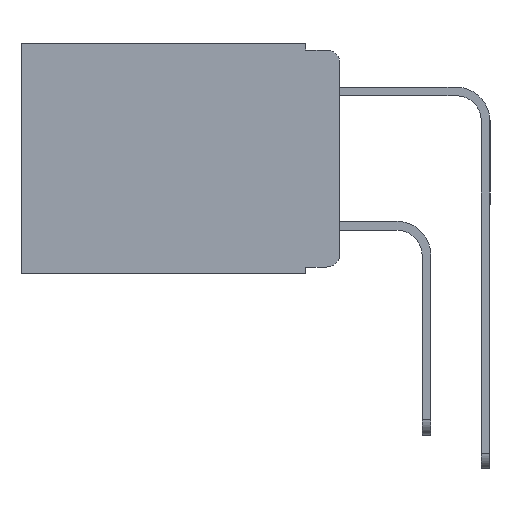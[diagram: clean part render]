
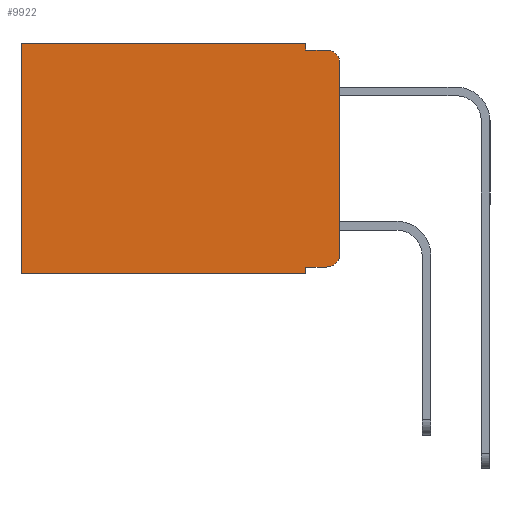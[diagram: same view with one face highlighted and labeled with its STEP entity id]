
A CAD part, left-side view. The second image highlights one B-rep face of the part: STEP entity #9922.
In plain terms, the highlighted planar face has unit normal (-1, 0, 0).
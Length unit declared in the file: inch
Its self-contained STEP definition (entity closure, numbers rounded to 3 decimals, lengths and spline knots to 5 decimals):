
#86 = DIRECTION ( 'NONE',  ( 0., -1., 0. ) ) ;
#463 = ORIENTED_EDGE ( 'NONE', *, *, #11980, .T. ) ;
#1903 = ORIENTED_EDGE ( 'NONE', *, *, #7288, .F. ) ;
#2414 = DIRECTION ( 'NONE',  ( 0., 1., 0. ) ) ;
#2755 = DIRECTION ( 'NONE',  ( 0., -1., 0. ) ) ;
#2843 = PLANE ( 'NONE',  #14372 ) ;
#3062 = VERTEX_POINT ( 'NONE', #25714 ) ;
#3733 = CARTESIAN_POINT ( 'NONE',  ( 0.298, 0.02, -0.01 ) ) ;
#3858 = CIRCLE ( 'NONE', #24096, 0.02 ) ;
#4235 = DIRECTION ( 'NONE',  ( -1., 0., 0. ) ) ;
#4253 = DIRECTION ( 'NONE',  ( 0., 1., 0. ) ) ;
#4342 = LINE ( 'NONE', #17061, #10380 ) ;
#4482 = ORIENTED_EDGE ( 'NONE', *, *, #24806, .T. ) ;
#4807 = CARTESIAN_POINT ( 'NONE',  ( 0.298, 0.051, -0.01 ) ) ;
#4888 = ORIENTED_EDGE ( 'NONE', *, *, #13880, .T. ) ;
#4929 = VERTEX_POINT ( 'NONE', #17429 ) ;
#4936 = ORIENTED_EDGE ( 'NONE', *, *, #9673, .T. ) ;
#5093 = CARTESIAN_POINT ( 'NONE',  ( 0.298, 0.473, -0.343 ) ) ;
#5241 = EDGE_CURVE ( 'NONE', #3062, #19628, #8568, .T. ) ;
#6162 = CARTESIAN_POINT ( 'NONE',  ( 0.298, 0.02, -0.313 ) ) ;
#6866 = ORIENTED_EDGE ( 'NONE', *, *, #23828, .F. ) ;
#6951 = DIRECTION ( 'NONE',  ( 1., 0., 0. ) ) ;
#7134 = DIRECTION ( 'NONE',  ( 0., 0., -1. ) ) ;
#7288 = EDGE_CURVE ( 'NONE', #14667, #13865, #4342, .T. ) ;
#7534 = VERTEX_POINT ( 'NONE', #9285 ) ;
#7767 = CARTESIAN_POINT ( 'NONE',  ( 0.298, 0., -0.03 ) ) ;
#7936 = VECTOR ( 'NONE', #2414, 39.37008 ) ;
#8239 = DIRECTION ( 'NONE',  ( 0., 0., -1. ) ) ;
#8568 = LINE ( 'NONE', #14480, #7936 ) ;
#8742 = ORIENTED_EDGE ( 'NONE', *, *, #5241, .F. ) ;
#9285 = CARTESIAN_POINT ( 'NONE',  ( 0.298, 0.02, -0.333 ) ) ;
#9466 = ORIENTED_EDGE ( 'NONE', *, *, #17623, .T. ) ;
#9596 = VECTOR ( 'NONE', #13378, 39.37008 ) ;
#9673 = EDGE_CURVE ( 'NONE', #17581, #7534, #11264, .T. ) ;
#9888 = EDGE_CURVE ( 'NONE', #13865, #25794, #21395, .T. ) ;
#9922 = ADVANCED_FACE ( 'NONE', ( #20783 ), #2843, .F. ) ;
#10220 = LINE ( 'NONE', #15357, #9596 ) ;
#10227 = VERTEX_POINT ( 'NONE', #13863 ) ;
#10302 = CARTESIAN_POINT ( 'NONE',  ( 0.298, 0.051, -0.01 ) ) ;
#10380 = VECTOR ( 'NONE', #7134, 39.37008 ) ;
#11264 = LINE ( 'NONE', #14222, #21714 ) ;
#11517 = VECTOR ( 'NONE', #12064, 39.37008 ) ;
#11980 = EDGE_CURVE ( 'NONE', #10227, #19628, #10220, .T. ) ;
#12064 = DIRECTION ( 'NONE',  ( 0., 0., -1. ) ) ;
#12316 = VECTOR ( 'NONE', #4253, 39.37008 ) ;
#13378 = DIRECTION ( 'NONE',  ( 0., 0., -1. ) ) ;
#13863 = CARTESIAN_POINT ( 'NONE',  ( 0.298, 0.473, 0. ) ) ;
#13865 = VERTEX_POINT ( 'NONE', #10302 ) ;
#13880 = EDGE_CURVE ( 'NONE', #14667, #10227, #17542, .T. ) ;
#14222 = CARTESIAN_POINT ( 'NONE',  ( 0.298, 0.051, -0.333 ) ) ;
#14372 = AXIS2_PLACEMENT_3D ( 'NONE', #18855, #6951, #20831 ) ;
#14480 = CARTESIAN_POINT ( 'NONE',  ( 0.298, 0., -0.343 ) ) ;
#14667 = VERTEX_POINT ( 'NONE', #18901 ) ;
#14931 = LINE ( 'NONE', #24824, #24759 ) ;
#15247 = ORIENTED_EDGE ( 'NONE', *, *, #9888, .F. ) ;
#15357 = CARTESIAN_POINT ( 'NONE',  ( 0.298, 0.473, 0. ) ) ;
#16180 = VECTOR ( 'NONE', #2755, 39.37008 ) ;
#16251 = CARTESIAN_POINT ( 'NONE',  ( 0.298, 0.02, -0.03 ) ) ;
#17061 = CARTESIAN_POINT ( 'NONE',  ( 0.298, 0.051, 0. ) ) ;
#17260 = EDGE_CURVE ( 'NONE', #18186, #4929, #14931, .T. ) ;
#17374 = CIRCLE ( 'NONE', #23993, 0.02 ) ;
#17429 = CARTESIAN_POINT ( 'NONE',  ( 0.298, 0., -0.313 ) ) ;
#17542 = LINE ( 'NONE', #22102, #12316 ) ;
#17581 = VERTEX_POINT ( 'NONE', #19922 ) ;
#17623 = EDGE_CURVE ( 'NONE', #7534, #4929, #17374, .T. ) ;
#18186 = VERTEX_POINT ( 'NONE', #7767 ) ;
#18215 = DIRECTION ( 'NONE',  ( 0., 0., -1. ) ) ;
#18660 = ORIENTED_EDGE ( 'NONE', *, *, #17260, .F. ) ;
#18855 = CARTESIAN_POINT ( 'NONE',  ( 0.298, 0., 0. ) ) ;
#18901 = CARTESIAN_POINT ( 'NONE',  ( 0.298, 0.051, 0. ) ) ;
#19628 = VERTEX_POINT ( 'NONE', #5093 ) ;
#19922 = CARTESIAN_POINT ( 'NONE',  ( 0.298, 0.051, -0.333 ) ) ;
#20078 = DIRECTION ( 'NONE',  ( -1., 0., 0. ) ) ;
#20783 = FACE_OUTER_BOUND ( 'NONE', #23558, .T. ) ;
#20831 = DIRECTION ( 'NONE',  ( 0., 0., -1. ) ) ;
#20880 = DIRECTION ( 'NONE',  ( 0., 0., -1. ) ) ;
#21395 = LINE ( 'NONE', #4807, #16180 ) ;
#21714 = VECTOR ( 'NONE', #86, 39.37008 ) ;
#21939 = CARTESIAN_POINT ( 'NONE',  ( 0.298, 0.051, 0. ) ) ;
#22102 = CARTESIAN_POINT ( 'NONE',  ( 0.298, 0., 0. ) ) ;
#22580 = LINE ( 'NONE', #21939, #11517 ) ;
#23558 = EDGE_LOOP ( 'NONE', ( #18660, #4482, #15247, #1903, #4888, #463, #8742, #6866, #4936, #9466 ) ) ;
#23828 = EDGE_CURVE ( 'NONE', #17581, #3062, #22580, .T. ) ;
#23993 = AXIS2_PLACEMENT_3D ( 'NONE', #6162, #20078, #8239 ) ;
#24096 = AXIS2_PLACEMENT_3D ( 'NONE', #16251, #4235, #18215 ) ;
#24759 = VECTOR ( 'NONE', #20880, 39.37008 ) ;
#24806 = EDGE_CURVE ( 'NONE', #18186, #25794, #3858, .T. ) ;
#24824 = CARTESIAN_POINT ( 'NONE',  ( 0.298, 0., 0. ) ) ;
#25714 = CARTESIAN_POINT ( 'NONE',  ( 0.298, 0.051, -0.343 ) ) ;
#25794 = VERTEX_POINT ( 'NONE', #3733 ) ;
